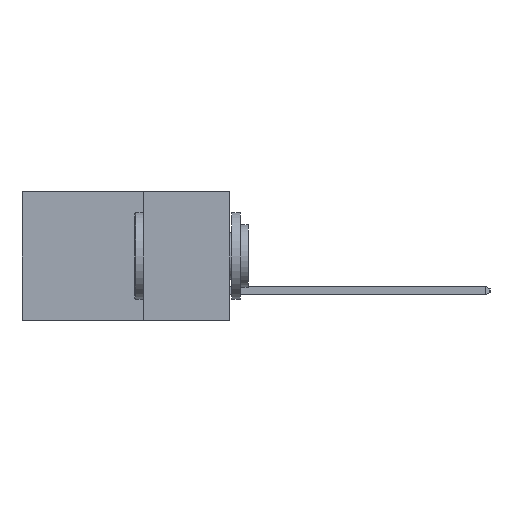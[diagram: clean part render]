
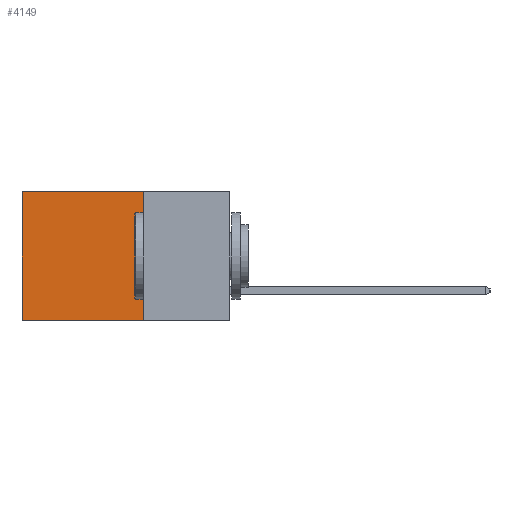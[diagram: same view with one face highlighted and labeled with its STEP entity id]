
A CAD part, left-side view. The second image highlights one B-rep face of the part: STEP entity #4149.
In plain terms, the highlighted planar face has unit normal (-1, 0, 0).
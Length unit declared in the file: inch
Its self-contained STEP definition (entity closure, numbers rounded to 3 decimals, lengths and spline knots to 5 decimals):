
#764 = ORIENTED_EDGE ( 'NONE', *, *, #6193, .T. ) ;
#862 = ORIENTED_EDGE ( 'NONE', *, *, #11583, .T. ) ;
#1619 = VECTOR ( 'NONE', #2663, 39.37008 ) ;
#1730 = ORIENTED_EDGE ( 'NONE', *, *, #5682, .F. ) ;
#2259 = VECTOR ( 'NONE', #9080, 39.37008 ) ;
#2281 = CARTESIAN_POINT ( 'NONE',  ( 0.2615, 0.25, 0. ) ) ;
#2564 = CARTESIAN_POINT ( 'NONE',  ( 0.2615, 0.25, -0.37 ) ) ;
#2663 = DIRECTION ( 'NONE',  ( 0., 0., -1. ) ) ;
#2678 = CARTESIAN_POINT ( 'NONE',  ( 0.2615, 0.6, -0.37 ) ) ;
#2701 = LINE ( 'NONE', #11685, #5193 ) ;
#2943 = DIRECTION ( 'NONE',  ( 0., 1., 0. ) ) ;
#3071 = VECTOR ( 'NONE', #2943, 39.37008 ) ;
#3417 = AXIS2_PLACEMENT_3D ( 'NONE', #4020, #3496, #3479 ) ;
#3423 = CARTESIAN_POINT ( 'NONE',  ( 0.2615, 0.25, -0.37 ) ) ;
#3479 = DIRECTION ( 'NONE',  ( 0., 0., -1. ) ) ;
#3496 = DIRECTION ( 'NONE',  ( 1., 0., 0. ) ) ;
#3636 = VERTEX_POINT ( 'NONE', #3738 ) ;
#3738 = CARTESIAN_POINT ( 'NONE',  ( 0.2615, 0.6, -0.37 ) ) ;
#4020 = CARTESIAN_POINT ( 'NONE',  ( 0.2615, 0.25, -0.37 ) ) ;
#4032 = PLANE ( 'NONE',  #3417 ) ;
#4149 = ADVANCED_FACE ( 'NONE', ( #10545 ), #4032, .F. ) ;
#4494 = ORIENTED_EDGE ( 'NONE', *, *, #11799, .F. ) ;
#5193 = VECTOR ( 'NONE', #11735, 39.37008 ) ;
#5423 = EDGE_LOOP ( 'NONE', ( #862, #4494, #1730, #764 ) ) ;
#5682 = EDGE_CURVE ( 'NONE', #9519, #6430, #8742, .T. ) ;
#6193 = EDGE_CURVE ( 'NONE', #9519, #7653, #2701, .T. ) ;
#6430 = VERTEX_POINT ( 'NONE', #2564 ) ;
#6581 = CARTESIAN_POINT ( 'NONE',  ( 0.2615, 0.25, -0.37 ) ) ;
#7181 = LINE ( 'NONE', #2678, #2259 ) ;
#7653 = VERTEX_POINT ( 'NONE', #9850 ) ;
#7952 = LINE ( 'NONE', #6581, #3071 ) ;
#8742 = LINE ( 'NONE', #3423, #1619 ) ;
#9080 = DIRECTION ( 'NONE',  ( 0., 0., -1. ) ) ;
#9519 = VERTEX_POINT ( 'NONE', #2281 ) ;
#9850 = CARTESIAN_POINT ( 'NONE',  ( 0.2615, 0.6, 0. ) ) ;
#10545 = FACE_OUTER_BOUND ( 'NONE', #5423, .T. ) ;
#11583 = EDGE_CURVE ( 'NONE', #7653, #3636, #7181, .T. ) ;
#11685 = CARTESIAN_POINT ( 'NONE',  ( 0.2615, 0.25, 0. ) ) ;
#11735 = DIRECTION ( 'NONE',  ( 0., 1., 0. ) ) ;
#11799 = EDGE_CURVE ( 'NONE', #6430, #3636, #7952, .T. ) ;
